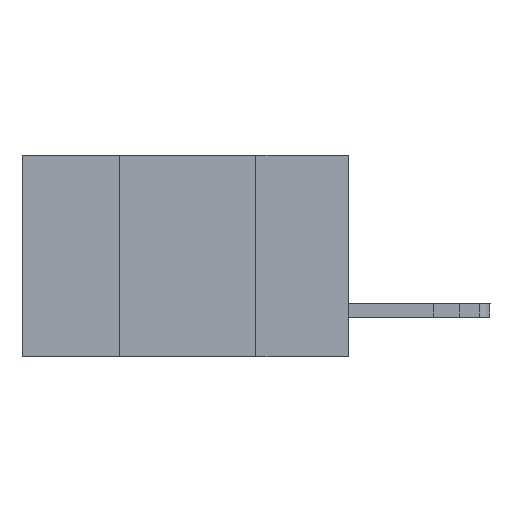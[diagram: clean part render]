
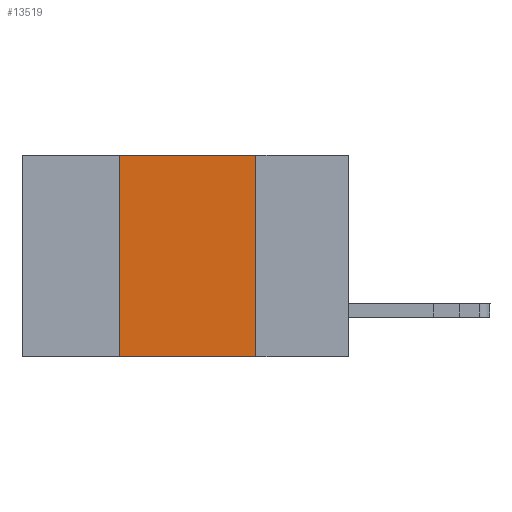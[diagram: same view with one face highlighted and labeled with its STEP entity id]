
A CAD part, left-side view. The second image highlights one B-rep face of the part: STEP entity #13519.
In plain terms, the highlighted planar face has unit normal (-1, 0, 0).
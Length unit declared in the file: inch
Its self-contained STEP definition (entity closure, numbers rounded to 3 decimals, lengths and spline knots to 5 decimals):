
#106 = EDGE_CURVE ( 'NONE', #6712, #15073, #18505, .T. ) ;
#258 = DIRECTION ( 'NONE',  ( 0., -1., 0. ) ) ;
#678 = CARTESIAN_POINT ( 'NONE',  ( 0., 0.6, 0. ) ) ;
#1199 = DIRECTION ( 'NONE',  ( 0., 0., -1. ) ) ;
#1474 = VECTOR ( 'NONE', #8449, 39.37008 ) ;
#2144 = ORIENTED_EDGE ( 'NONE', *, *, #11362, .T. ) ;
#2627 = LINE ( 'NONE', #15957, #1474 ) ;
#3314 = VERTEX_POINT ( 'NONE', #11823 ) ;
#3418 = VECTOR ( 'NONE', #258, 39.37008 ) ;
#3687 = CARTESIAN_POINT ( 'NONE',  ( 0., 0.42, -0.37 ) ) ;
#4565 = CARTESIAN_POINT ( 'NONE',  ( 0., 0.6, -0.37 ) ) ;
#4602 = ORIENTED_EDGE ( 'NONE', *, *, #106, .F. ) ;
#6666 = DIRECTION ( 'NONE',  ( 1., 0., 0. ) ) ;
#6712 = VERTEX_POINT ( 'NONE', #10850 ) ;
#7170 = VERTEX_POINT ( 'NONE', #3687 ) ;
#7327 = DIRECTION ( 'NONE',  ( 0., -1., 0. ) ) ;
#8169 = FACE_OUTER_BOUND ( 'NONE', #13785, .T. ) ;
#8449 = DIRECTION ( 'NONE',  ( 0., 0., 1. ) ) ;
#8683 = ORIENTED_EDGE ( 'NONE', *, *, #16278, .F. ) ;
#9035 = CARTESIAN_POINT ( 'NONE',  ( 0., 0.6, 0. ) ) ;
#9182 = AXIS2_PLACEMENT_3D ( 'NONE', #678, #6666, #12712 ) ;
#9876 = VECTOR ( 'NONE', #7327, 39.37008 ) ;
#10850 = CARTESIAN_POINT ( 'NONE',  ( 0., 0.42, 0. ) ) ;
#11160 = EDGE_CURVE ( 'NONE', #7170, #6712, #2627, .T. ) ;
#11362 = EDGE_CURVE ( 'NONE', #7170, #3314, #12091, .T. ) ;
#11823 = CARTESIAN_POINT ( 'NONE',  ( 0., 0.17, -0.37 ) ) ;
#12072 = ORIENTED_EDGE ( 'NONE', *, *, #11160, .F. ) ;
#12091 = LINE ( 'NONE', #4565, #9876 ) ;
#12712 = DIRECTION ( 'NONE',  ( 0., 0., -1. ) ) ;
#13519 = ADVANCED_FACE ( 'NONE', ( #8169 ), #14185, .F. ) ;
#13785 = EDGE_LOOP ( 'NONE', ( #8683, #4602, #12072, #2144 ) ) ;
#14185 = PLANE ( 'NONE',  #9182 ) ;
#14305 = VECTOR ( 'NONE', #1199, 39.37008 ) ;
#14703 = CARTESIAN_POINT ( 'NONE',  ( 0., 0.17, -0.37 ) ) ;
#15073 = VERTEX_POINT ( 'NONE', #18116 ) ;
#15957 = CARTESIAN_POINT ( 'NONE',  ( 0., 0.42, -0.37 ) ) ;
#16278 = EDGE_CURVE ( 'NONE', #15073, #3314, #19155, .T. ) ;
#18116 = CARTESIAN_POINT ( 'NONE',  ( 0., 0.17, 0. ) ) ;
#18505 = LINE ( 'NONE', #9035, #3418 ) ;
#19155 = LINE ( 'NONE', #14703, #14305 ) ;
